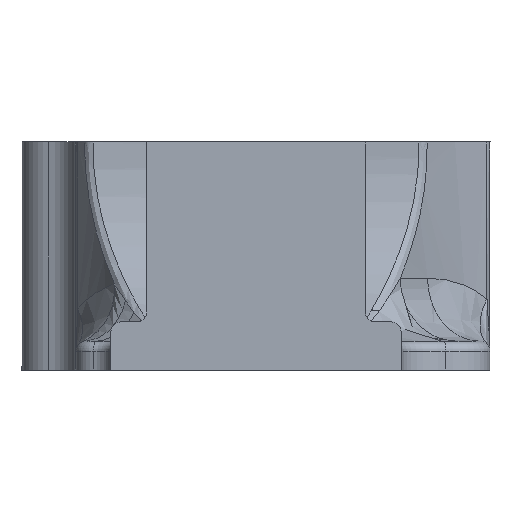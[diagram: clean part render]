
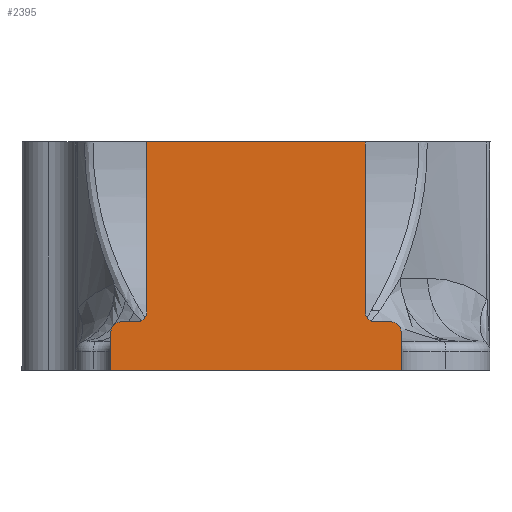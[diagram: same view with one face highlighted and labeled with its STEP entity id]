
A CAD part, front view. The second image highlights one B-rep face of the part: STEP entity #2395.
In plain terms, the highlighted planar face has unit normal (0, -1, 0).
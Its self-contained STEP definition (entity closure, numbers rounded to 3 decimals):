
#15 = EDGE_LOOP ( 'NONE', ( #1345, #1077, #5395, #2489, #2814, #3482, #1362, #1303, #4191, #2124, #1321, #3100 ) ) ;
#280 = VERTEX_POINT ( 'NONE', #1318 ) ;
#333 = EDGE_CURVE ( 'NONE', #2787, #2968, #2360, .T. ) ;
#361 = EDGE_CURVE ( 'NONE', #387, #3503, #4184, .T. ) ;
#370 = EDGE_CURVE ( 'NONE', #4441, #1338, #974, .T. ) ;
#387 = VERTEX_POINT ( 'NONE', #4569 ) ;
#396 = EDGE_CURVE ( 'NONE', #1215, #280, #4451, .T. ) ;
#407 = CARTESIAN_POINT ( 'NONE',  ( 4.067, -36.122, 209.248 ) ) ;
#421 = CARTESIAN_POINT ( 'NONE',  ( 3.273, -36.122, 209.248 ) ) ;
#583 = VECTOR ( 'NONE', #3717, 1000. ) ;
#628 = EDGE_CURVE ( 'NONE', #1338, #3503, #2556, .T. ) ;
#707 = CARTESIAN_POINT ( 'NONE',  ( 24.225, -36.122, 204.645 ) ) ;
#817 = LINE ( 'NONE', #1138, #2932 ) ;
#844 = DIRECTION ( 'NONE',  ( 1., 0., 0. ) ) ;
#882 = DIRECTION ( 'NONE',  ( 0., 0., -1. ) ) ;
#941 = DIRECTION ( 'NONE',  ( 0., 1., 0. ) ) ;
#974 = CIRCLE ( 'NONE', #4992, 0.794 ) ;
#1043 = CARTESIAN_POINT ( 'NONE',  ( 4.067, -36.122, 222.736 ) ) ;
#1064 = VERTEX_POINT ( 'NONE', #707 ) ;
#1077 = ORIENTED_EDGE ( 'NONE', *, *, #5283, .F. ) ;
#1138 = CARTESIAN_POINT ( 'NONE',  ( 1.206, -36.122, 179.257 ) ) ;
#1154 = FACE_OUTER_BOUND ( 'NONE', #15, .T. ) ;
#1192 = PLANE ( 'NONE',  #2923 ) ;
#1215 = VERTEX_POINT ( 'NONE', #4038 ) ;
#1270 = VERTEX_POINT ( 'NONE', #1937 ) ;
#1303 = ORIENTED_EDGE ( 'NONE', *, *, #370, .T. ) ;
#1305 = CARTESIAN_POINT ( 'NONE',  ( 21.364, -36.122, 179.257 ) ) ;
#1318 = CARTESIAN_POINT ( 'NONE',  ( 1.206, -36.122, 207.661 ) ) ;
#1321 = ORIENTED_EDGE ( 'NONE', *, *, #2738, .T. ) ;
#1338 = VERTEX_POINT ( 'NONE', #4219 ) ;
#1345 = ORIENTED_EDGE ( 'NONE', *, *, #333, .F. ) ;
#1362 = ORIENTED_EDGE ( 'NONE', *, *, #5183, .F. ) ;
#1380 = EDGE_CURVE ( 'NONE', #1451, #1215, #1671, .T. ) ;
#1451 = VERTEX_POINT ( 'NONE', #2553 ) ;
#1544 = DIRECTION ( 'NONE',  ( 1., 0., 0. ) ) ;
#1563 = DIRECTION ( 'NONE',  ( 0., 0., -1. ) ) ;
#1636 = DIRECTION ( 'NONE',  ( 0., 0., 1. ) ) ;
#1671 = LINE ( 'NONE', #3766, #583 ) ;
#1812 = AXIS2_PLACEMENT_3D ( 'NONE', #421, #3360, #844 ) ;
#1937 = CARTESIAN_POINT ( 'NONE',  ( 21.364, -36.122, 222.736 ) ) ;
#1994 = LINE ( 'NONE', #4104, #5063 ) ;
#2052 = LINE ( 'NONE', #2834, #4036 ) ;
#2124 = ORIENTED_EDGE ( 'NONE', *, *, #361, .F. ) ;
#2220 = VECTOR ( 'NONE', #5377, 1000. ) ;
#2321 = DIRECTION ( 'NONE',  ( -1., 0., 0. ) ) ;
#2360 = LINE ( 'NONE', #5222, #2220 ) ;
#2395 = ADVANCED_FACE ( 'NONE', ( #1154 ), #1192, .F. ) ;
#2423 = VECTOR ( 'NONE', #2321, 1000. ) ;
#2489 = ORIENTED_EDGE ( 'NONE', *, *, #396, .T. ) ;
#2553 = CARTESIAN_POINT ( 'NONE',  ( 3.273, -36.122, 208.455 ) ) ;
#2556 = LINE ( 'NONE', #2762, #2423 ) ;
#2738 = EDGE_CURVE ( 'NONE', #387, #1270, #2885, .T. ) ;
#2762 = CARTESIAN_POINT ( 'NONE',  ( 24.225, -36.122, 208.455 ) ) ;
#2770 = LINE ( 'NONE', #4070, #5282 ) ;
#2782 = VERTEX_POINT ( 'NONE', #5408 ) ;
#2787 = VERTEX_POINT ( 'NONE', #407 ) ;
#2804 = CARTESIAN_POINT ( 'NONE',  ( 22.158, -36.122, 208.455 ) ) ;
#2814 = ORIENTED_EDGE ( 'NONE', *, *, #4553, .T. ) ;
#2834 = CARTESIAN_POINT ( 'NONE',  ( 24.225, -36.122, 179.257 ) ) ;
#2885 = LINE ( 'NONE', #4564, #3860 ) ;
#2923 = AXIS2_PLACEMENT_3D ( 'NONE', #1305, #941, #882 ) ;
#2932 = VECTOR ( 'NONE', #1563, 1000. ) ;
#2968 = VERTEX_POINT ( 'NONE', #1043 ) ;
#2973 = CARTESIAN_POINT ( 'NONE',  ( 24.225, -36.122, 207.661 ) ) ;
#3100 = ORIENTED_EDGE ( 'NONE', *, *, #3379, .F. ) ;
#3232 = DIRECTION ( 'NONE',  ( 0., 0., -1. ) ) ;
#3360 = DIRECTION ( 'NONE',  ( 0., -1., 0. ) ) ;
#3379 = EDGE_CURVE ( 'NONE', #2968, #1270, #2770, .T. ) ;
#3482 = ORIENTED_EDGE ( 'NONE', *, *, #4382, .T. ) ;
#3503 = VERTEX_POINT ( 'NONE', #2804 ) ;
#3676 = AXIS2_PLACEMENT_3D ( 'NONE', #4468, #4411, #4416 ) ;
#3714 = AXIS2_PLACEMENT_3D ( 'NONE', #4619, #4716, #4700 ) ;
#3717 = DIRECTION ( 'NONE',  ( -1., 0., 0. ) ) ;
#3766 = CARTESIAN_POINT ( 'NONE',  ( 24.225, -36.122, 208.455 ) ) ;
#3768 = CIRCLE ( 'NONE', #1812, 0.794 ) ;
#3770 = DIRECTION ( 'NONE',  ( 1., 0., 0. ) ) ;
#3860 = VECTOR ( 'NONE', #1636, 1000. ) ;
#4036 = VECTOR ( 'NONE', #3232, 1000. ) ;
#4038 = CARTESIAN_POINT ( 'NONE',  ( 2., -36.122, 208.455 ) ) ;
#4070 = CARTESIAN_POINT ( 'NONE',  ( -9.788, -36.122, 222.736 ) ) ;
#4104 = CARTESIAN_POINT ( 'NONE',  ( -9.788, -36.122, 204.645 ) ) ;
#4184 = CIRCLE ( 'NONE', #3714, 0.794 ) ;
#4191 = ORIENTED_EDGE ( 'NONE', *, *, #628, .T. ) ;
#4219 = CARTESIAN_POINT ( 'NONE',  ( 23.431, -36.122, 208.455 ) ) ;
#4382 = EDGE_CURVE ( 'NONE', #2782, #1064, #1994, .T. ) ;
#4411 = DIRECTION ( 'NONE',  ( 0., -1., 0. ) ) ;
#4416 = DIRECTION ( 'NONE',  ( 1., 0., 0. ) ) ;
#4441 = VERTEX_POINT ( 'NONE', #2973 ) ;
#4451 = CIRCLE ( 'NONE', #3676, 0.794 ) ;
#4468 = CARTESIAN_POINT ( 'NONE',  ( 2., -36.122, 207.661 ) ) ;
#4519 = CARTESIAN_POINT ( 'NONE',  ( 23.431, -36.122, 207.661 ) ) ;
#4552 = DIRECTION ( 'NONE',  ( 1., 0., 0. ) ) ;
#4553 = EDGE_CURVE ( 'NONE', #280, #2782, #817, .T. ) ;
#4564 = CARTESIAN_POINT ( 'NONE',  ( 21.364, -36.122, 179.257 ) ) ;
#4569 = CARTESIAN_POINT ( 'NONE',  ( 21.364, -36.122, 209.248 ) ) ;
#4587 = DIRECTION ( 'NONE',  ( 0., -1., 0. ) ) ;
#4619 = CARTESIAN_POINT ( 'NONE',  ( 22.158, -36.122, 209.248 ) ) ;
#4700 = DIRECTION ( 'NONE',  ( 1., 0., 0. ) ) ;
#4716 = DIRECTION ( 'NONE',  ( 0., -1., 0. ) ) ;
#4992 = AXIS2_PLACEMENT_3D ( 'NONE', #4519, #4587, #4552 ) ;
#5063 = VECTOR ( 'NONE', #3770, 1000. ) ;
#5183 = EDGE_CURVE ( 'NONE', #4441, #1064, #2052, .T. ) ;
#5222 = CARTESIAN_POINT ( 'NONE',  ( 4.067, -36.122, 179.257 ) ) ;
#5282 = VECTOR ( 'NONE', #1544, 1000. ) ;
#5283 = EDGE_CURVE ( 'NONE', #1451, #2787, #3768, .T. ) ;
#5377 = DIRECTION ( 'NONE',  ( 0., 0., 1. ) ) ;
#5395 = ORIENTED_EDGE ( 'NONE', *, *, #1380, .T. ) ;
#5408 = CARTESIAN_POINT ( 'NONE',  ( 1.206, -36.122, 204.645 ) ) ;
